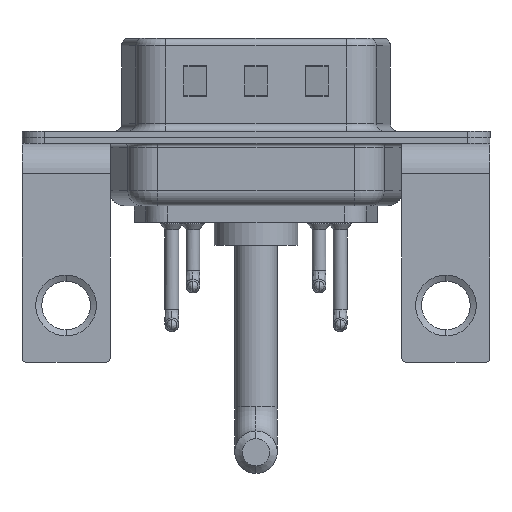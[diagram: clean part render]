
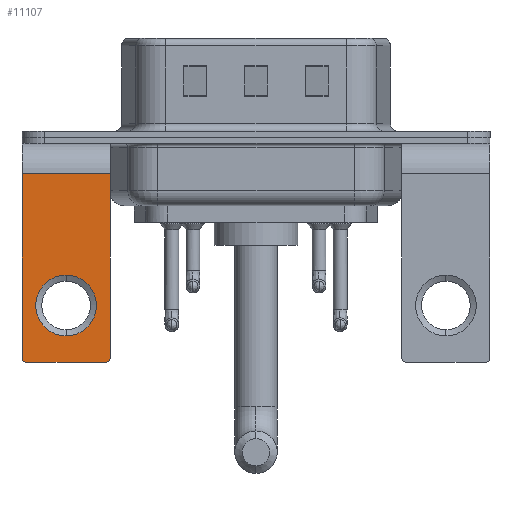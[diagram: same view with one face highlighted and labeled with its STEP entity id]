
A CAD part, front view. The second image highlights one B-rep face of the part: STEP entity #11107.
In plain terms, the highlighted planar face has unit normal (0, -1, 0).
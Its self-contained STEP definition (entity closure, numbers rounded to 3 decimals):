
#119 = CIRCLE ( 'NONE', #7309, 0.25 ) ;
#1425 = DIRECTION ( 'NONE',  ( 0., 0., 1. ) ) ;
#1501 = VECTOR ( 'NONE', #17121, 1000. ) ;
#2334 = EDGE_CURVE ( 'NONE', #15486, #6166, #7605, .T. ) ;
#2422 = AXIS2_PLACEMENT_3D ( 'NONE', #10139, #8599, #14871 ) ;
#2501 = EDGE_CURVE ( 'NONE', #15248, #6166, #13663, .T. ) ;
#2546 = DIRECTION ( 'NONE',  ( 0., 1., 0. ) ) ;
#2700 = CARTESIAN_POINT ( 'NONE',  ( -2.9, -6.25, -14.55 ) ) ;
#2815 = CARTESIAN_POINT ( 'NONE',  ( 2.9, -6.25, -14.55 ) ) ;
#3229 = LINE ( 'NONE', #15767, #11706 ) ;
#3271 = DIRECTION ( 'NONE',  ( -1., 0., 0. ) ) ;
#3423 = CARTESIAN_POINT ( 'NONE',  ( 2.65, -6.25, -14.8 ) ) ;
#4310 = FACE_BOUND ( 'NONE', #4971, .T. ) ;
#4671 = CARTESIAN_POINT ( 'NONE',  ( 0., -6.25, -13.07 ) ) ;
#4939 = EDGE_CURVE ( 'NONE', #10049, #16451, #7449, .T. ) ;
#4971 = EDGE_LOOP ( 'NONE', ( #15288, #9613 ) ) ;
#5326 = ORIENTED_EDGE ( 'NONE', *, *, #2334, .T. ) ;
#5419 = ORIENTED_EDGE ( 'NONE', *, *, #14712, .T. ) ;
#5555 = DIRECTION ( 'NONE',  ( 0., 0., 1. ) ) ;
#6132 = FACE_OUTER_BOUND ( 'NONE', #9670, .T. ) ;
#6166 = VERTEX_POINT ( 'NONE', #16413 ) ;
#6643 = DIRECTION ( 'NONE',  ( -1., 0., 0. ) ) ;
#7309 = AXIS2_PLACEMENT_3D ( 'NONE', #12704, #19371, #12805 ) ;
#7342 = VECTOR ( 'NONE', #13923, 1000. ) ;
#7449 = LINE ( 'NONE', #13724, #1501 ) ;
#7605 = CIRCLE ( 'NONE', #19090, 0.25 ) ;
#7698 = ORIENTED_EDGE ( 'NONE', *, *, #4939, .F. ) ;
#8166 = EDGE_CURVE ( 'NONE', #10049, #10522, #3229, .T. ) ;
#8478 = VERTEX_POINT ( 'NONE', #16169 ) ;
#8599 = DIRECTION ( 'NONE',  ( 0., 1., 0. ) ) ;
#8719 = AXIS2_PLACEMENT_3D ( 'NONE', #13841, #12423, #1425 ) ;
#9233 = EDGE_CURVE ( 'NONE', #8478, #13697, #11280, .T. ) ;
#9265 = ORIENTED_EDGE ( 'NONE', *, *, #8166, .T. ) ;
#9344 = EDGE_CURVE ( 'NONE', #10522, #15486, #10338, .T. ) ;
#9611 = VECTOR ( 'NONE', #3271, 1000. ) ;
#9613 = ORIENTED_EDGE ( 'NONE', *, *, #9233, .T. ) ;
#9651 = ORIENTED_EDGE ( 'NONE', *, *, #9344, .T. ) ;
#9670 = EDGE_LOOP ( 'NONE', ( #9651, #5326, #13647, #5419, #7698, #9265 ) ) ;
#9987 = CARTESIAN_POINT ( 'NONE',  ( 2.9, -6.25, -2.4 ) ) ;
#10049 = VERTEX_POINT ( 'NONE', #9987 ) ;
#10139 = CARTESIAN_POINT ( 'NONE',  ( 0., -6.25, -11.07 ) ) ;
#10338 = LINE ( 'NONE', #16615, #7342 ) ;
#10522 = VERTEX_POINT ( 'NONE', #19516 ) ;
#11107 = ADVANCED_FACE ( 'NONE', ( #4310, #6132 ), #17139, .F. ) ;
#11280 = CIRCLE ( 'NONE', #2422, 2. ) ;
#11706 = VECTOR ( 'NONE', #6643, 1000. ) ;
#12040 = CARTESIAN_POINT ( 'NONE',  ( 2.9, -6.25, -14.8 ) ) ;
#12423 = DIRECTION ( 'NONE',  ( 0., 1., 0. ) ) ;
#12704 = CARTESIAN_POINT ( 'NONE',  ( 2.65, -6.25, -14.55 ) ) ;
#12805 = DIRECTION ( 'NONE',  ( 0., 0., 1. ) ) ;
#13164 = CARTESIAN_POINT ( 'NONE',  ( -2.65, -6.25, -14.55 ) ) ;
#13530 = DIRECTION ( 'NONE',  ( 0., 0., 1. ) ) ;
#13647 = ORIENTED_EDGE ( 'NONE', *, *, #2501, .F. ) ;
#13663 = LINE ( 'NONE', #12040, #9611 ) ;
#13697 = VERTEX_POINT ( 'NONE', #4671 ) ;
#13724 = CARTESIAN_POINT ( 'NONE',  ( 2.9, -6.25, -2.4 ) ) ;
#13841 = CARTESIAN_POINT ( 'NONE',  ( 2.9, -6.25, -2.4 ) ) ;
#13923 = DIRECTION ( 'NONE',  ( 0., 0., -1. ) ) ;
#14712 = EDGE_CURVE ( 'NONE', #15248, #16451, #119, .T. ) ;
#14871 = DIRECTION ( 'NONE',  ( 0., 0., 1. ) ) ;
#15183 = CARTESIAN_POINT ( 'NONE',  ( 0., -6.25, -11.07 ) ) ;
#15248 = VERTEX_POINT ( 'NONE', #3423 ) ;
#15288 = ORIENTED_EDGE ( 'NONE', *, *, #19720, .T. ) ;
#15486 = VERTEX_POINT ( 'NONE', #2700 ) ;
#15740 = AXIS2_PLACEMENT_3D ( 'NONE', #15183, #2546, #13530 ) ;
#15767 = CARTESIAN_POINT ( 'NONE',  ( 2.9, -6.25, -2.4 ) ) ;
#16169 = CARTESIAN_POINT ( 'NONE',  ( 0., -6.25, -9.07 ) ) ;
#16242 = DIRECTION ( 'NONE',  ( 0., -1., 0. ) ) ;
#16413 = CARTESIAN_POINT ( 'NONE',  ( -2.65, -6.25, -14.8 ) ) ;
#16451 = VERTEX_POINT ( 'NONE', #2815 ) ;
#16615 = CARTESIAN_POINT ( 'NONE',  ( -2.9, -6.25, -2.4 ) ) ;
#16728 = CIRCLE ( 'NONE', #15740, 2. ) ;
#17121 = DIRECTION ( 'NONE',  ( 0., 0., -1. ) ) ;
#17139 = PLANE ( 'NONE',  #8719 ) ;
#19090 = AXIS2_PLACEMENT_3D ( 'NONE', #13164, #16242, #5555 ) ;
#19371 = DIRECTION ( 'NONE',  ( 0., -1., 0. ) ) ;
#19516 = CARTESIAN_POINT ( 'NONE',  ( -2.9, -6.25, -2.4 ) ) ;
#19720 = EDGE_CURVE ( 'NONE', #13697, #8478, #16728, .T. ) ;
